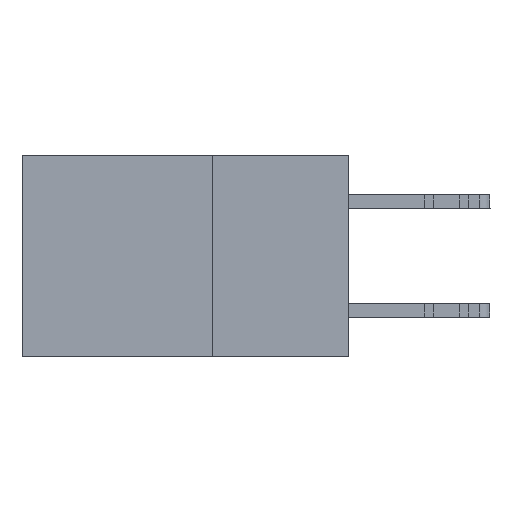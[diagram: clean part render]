
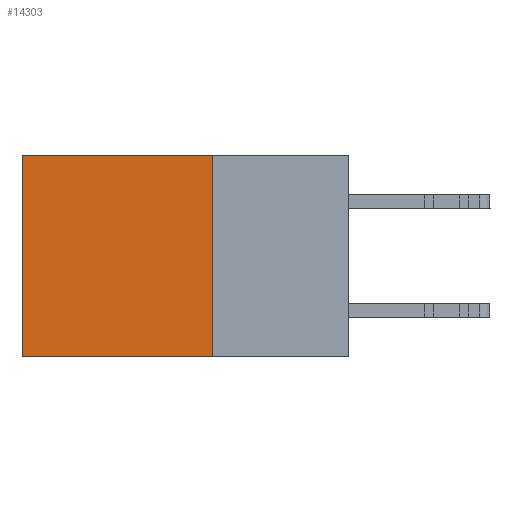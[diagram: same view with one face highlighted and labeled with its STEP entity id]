
A CAD part, left-side view. The second image highlights one B-rep face of the part: STEP entity #14303.
In plain terms, the highlighted planar face has unit normal (-1, 0, 0).
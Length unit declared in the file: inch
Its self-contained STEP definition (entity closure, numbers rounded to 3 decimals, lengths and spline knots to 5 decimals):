
#370 = VERTEX_POINT ( 'NONE', #9701 ) ;
#1114 = LINE ( 'NONE', #17461, #8240 ) ;
#1235 = DIRECTION ( 'NONE',  ( 0., 1., 0. ) ) ;
#1577 = VERTEX_POINT ( 'NONE', #3227 ) ;
#1921 = EDGE_LOOP ( 'NONE', ( #21314, #5769, #22650, #3139 ) ) ;
#2045 = LINE ( 'NONE', #5360, #15478 ) ;
#3139 = ORIENTED_EDGE ( 'NONE', *, *, #13565, .T. ) ;
#3227 = CARTESIAN_POINT ( 'NONE',  ( 0.2615, 0.6, -0.37 ) ) ;
#4204 = CARTESIAN_POINT ( 'NONE',  ( 0.2615, 0.25, -0.37 ) ) ;
#4674 = DIRECTION ( 'NONE',  ( 0., 0., -1. ) ) ;
#5360 = CARTESIAN_POINT ( 'NONE',  ( 0.2615, 0.6, -0.37 ) ) ;
#5504 = VECTOR ( 'NONE', #17393, 39.37008 ) ;
#5589 = DIRECTION ( 'NONE',  ( 0., 0., -1. ) ) ;
#5769 = ORIENTED_EDGE ( 'NONE', *, *, #18970, .F. ) ;
#6994 = VECTOR ( 'NONE', #4674, 39.37008 ) ;
#7693 = EDGE_CURVE ( 'NONE', #9158, #370, #9872, .T. ) ;
#8137 = AXIS2_PLACEMENT_3D ( 'NONE', #4204, #17098, #21983 ) ;
#8240 = VECTOR ( 'NONE', #1235, 39.37008 ) ;
#9158 = VERTEX_POINT ( 'NONE', #23037 ) ;
#9701 = CARTESIAN_POINT ( 'NONE',  ( 0.2615, 0.25, -0.37 ) ) ;
#9868 = PLANE ( 'NONE',  #8137 ) ;
#9872 = LINE ( 'NONE', #17102, #6994 ) ;
#10824 = EDGE_CURVE ( 'NONE', #21356, #1577, #2045, .T. ) ;
#13565 = EDGE_CURVE ( 'NONE', #9158, #21356, #19180, .T. ) ;
#14303 = ADVANCED_FACE ( 'NONE', ( #15006 ), #9868, .F. ) ;
#15006 = FACE_OUTER_BOUND ( 'NONE', #1921, .T. ) ;
#15478 = VECTOR ( 'NONE', #5589, 39.37008 ) ;
#17098 = DIRECTION ( 'NONE',  ( 1., 0., 0. ) ) ;
#17102 = CARTESIAN_POINT ( 'NONE',  ( 0.2615, 0.25, -0.37 ) ) ;
#17393 = DIRECTION ( 'NONE',  ( 0., 1., 0. ) ) ;
#17461 = CARTESIAN_POINT ( 'NONE',  ( 0.2615, 0.25, -0.37 ) ) ;
#18970 = EDGE_CURVE ( 'NONE', #370, #1577, #1114, .T. ) ;
#19180 = LINE ( 'NONE', #22851, #5504 ) ;
#21314 = ORIENTED_EDGE ( 'NONE', *, *, #10824, .T. ) ;
#21356 = VERTEX_POINT ( 'NONE', #22865 ) ;
#21983 = DIRECTION ( 'NONE',  ( 0., 0., -1. ) ) ;
#22650 = ORIENTED_EDGE ( 'NONE', *, *, #7693, .F. ) ;
#22851 = CARTESIAN_POINT ( 'NONE',  ( 0.2615, 0.25, 0. ) ) ;
#22865 = CARTESIAN_POINT ( 'NONE',  ( 0.2615, 0.6, 0. ) ) ;
#23037 = CARTESIAN_POINT ( 'NONE',  ( 0.2615, 0.25, 0. ) ) ;
